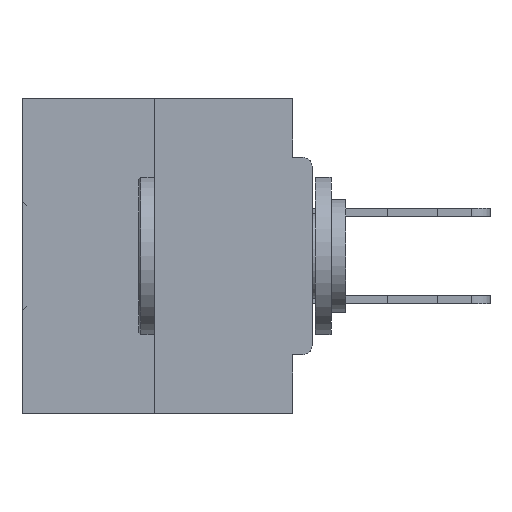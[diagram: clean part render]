
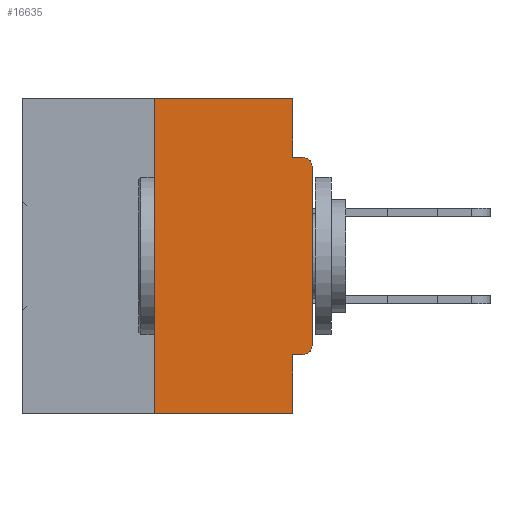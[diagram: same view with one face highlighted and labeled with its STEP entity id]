
A CAD part, left-side view. The second image highlights one B-rep face of the part: STEP entity #16635.
In plain terms, the highlighted planar face has unit normal (-1, 0, 0).
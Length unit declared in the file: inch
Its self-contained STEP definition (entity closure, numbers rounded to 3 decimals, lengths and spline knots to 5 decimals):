
#239 = VERTEX_POINT ( 'NONE', #18586 ) ;
#442 = VECTOR ( 'NONE', #19045, 39.37008 ) ;
#1625 = FACE_OUTER_BOUND ( 'NONE', #19300, .T. ) ;
#1790 = DIRECTION ( 'NONE',  ( 0., -1., 0. ) ) ;
#2994 = DIRECTION ( 'NONE',  ( 0., -1., 0. ) ) ;
#3037 = ORIENTED_EDGE ( 'NONE', *, *, #3227, .T. ) ;
#3147 = CARTESIAN_POINT ( 'NONE',  ( 0., 0.015, -0.4065 ) ) ;
#3227 = EDGE_CURVE ( 'NONE', #5612, #7826, #10813, .T. ) ;
#3352 = VECTOR ( 'NONE', #39458, 39.37008 ) ;
#4284 = CARTESIAN_POINT ( 'NONE',  ( 0., 0.25, 0. ) ) ;
#4488 = CARTESIAN_POINT ( 'NONE',  ( 0., 0.25, -0.5 ) ) ;
#4504 = LINE ( 'NONE', #40406, #442 ) ;
#4507 = AXIS2_PLACEMENT_3D ( 'NONE', #10167, #28764, #24775 ) ;
#5444 = LINE ( 'NONE', #20896, #45046 ) ;
#5584 = ORIENTED_EDGE ( 'NONE', *, *, #29936, .T. ) ;
#5612 = VERTEX_POINT ( 'NONE', #4488 ) ;
#6881 = LINE ( 'NONE', #23424, #43581 ) ;
#7826 = VERTEX_POINT ( 'NONE', #43231 ) ;
#8266 = ORIENTED_EDGE ( 'NONE', *, *, #36884, .T. ) ;
#9580 = VECTOR ( 'NONE', #22612, 39.37008 ) ;
#10167 = CARTESIAN_POINT ( 'NONE',  ( 0., 0.46, 0. ) ) ;
#10813 = LINE ( 'NONE', #12649, #36668 ) ;
#12649 = CARTESIAN_POINT ( 'NONE',  ( 0., 0.46, -0.5 ) ) ;
#12900 = VERTEX_POINT ( 'NONE', #28956 ) ;
#15367 = CARTESIAN_POINT ( 'NONE',  ( 0., 0.031, -0.5 ) ) ;
#16208 = LINE ( 'NONE', #46925, #29910 ) ;
#16635 = ADVANCED_FACE ( 'NONE', ( #1625 ), #39859, .F. ) ;
#17139 = CARTESIAN_POINT ( 'NONE',  ( 0., 0., -0.1085 ) ) ;
#17204 = AXIS2_PLACEMENT_3D ( 'NONE', #42694, #28243, #31471 ) ;
#18361 = DIRECTION ( 'NONE',  ( 0., 0., -1. ) ) ;
#18586 = CARTESIAN_POINT ( 'NONE',  ( 0., 0., -0.3915 ) ) ;
#19045 = DIRECTION ( 'NONE',  ( 0., 0., 1. ) ) ;
#19300 = EDGE_LOOP ( 'NONE', ( #36694, #38656, #3037, #40947, #28235, #27620, #5584, #8266, #20617, #40931 ) ) ;
#20617 = ORIENTED_EDGE ( 'NONE', *, *, #46822, .F. ) ;
#20896 = CARTESIAN_POINT ( 'NONE',  ( 0., 0.25, 0. ) ) ;
#21068 = CARTESIAN_POINT ( 'NONE',  ( 0., 0.031, -0.4065 ) ) ;
#22298 = CIRCLE ( 'NONE', #34668, 0.015 ) ;
#22612 = DIRECTION ( 'NONE',  ( 0., 0., -1. ) ) ;
#23424 = CARTESIAN_POINT ( 'NONE',  ( 0., 0., -0.0935 ) ) ;
#24067 = DIRECTION ( 'NONE',  ( 0., -1., 0. ) ) ;
#24616 = EDGE_CURVE ( 'NONE', #45241, #7826, #30230, .T. ) ;
#24775 = DIRECTION ( 'NONE',  ( 0., 0., -1. ) ) ;
#27364 = EDGE_CURVE ( 'NONE', #33543, #47430, #16208, .T. ) ;
#27620 = ORIENTED_EDGE ( 'NONE', *, *, #30322, .T. ) ;
#28095 = VERTEX_POINT ( 'NONE', #17139 ) ;
#28235 = ORIENTED_EDGE ( 'NONE', *, *, #29816, .F. ) ;
#28243 = DIRECTION ( 'NONE',  ( -1., 0., 0. ) ) ;
#28764 = DIRECTION ( 'NONE',  ( 1., 0., 0. ) ) ;
#28956 = CARTESIAN_POINT ( 'NONE',  ( 0., 0.015, -0.0935 ) ) ;
#29210 = VERTEX_POINT ( 'NONE', #3147 ) ;
#29816 = EDGE_CURVE ( 'NONE', #29210, #45241, #44090, .T. ) ;
#29910 = VECTOR ( 'NONE', #2994, 39.37008 ) ;
#29936 = EDGE_CURVE ( 'NONE', #239, #28095, #4504, .T. ) ;
#30230 = LINE ( 'NONE', #15367, #9580 ) ;
#30322 = EDGE_CURVE ( 'NONE', #29210, #239, #41180, .T. ) ;
#31388 = LINE ( 'NONE', #34684, #38308 ) ;
#31471 = DIRECTION ( 'NONE',  ( 0., 0., -1. ) ) ;
#31506 = DIRECTION ( 'NONE',  ( 0., 0., 1. ) ) ;
#32806 = EDGE_CURVE ( 'NONE', #5612, #33543, #5444, .T. ) ;
#32844 = CARTESIAN_POINT ( 'NONE',  ( 0., 0.015, -0.1085 ) ) ;
#33318 = DIRECTION ( 'NONE',  ( -1., 0., 0. ) ) ;
#33543 = VERTEX_POINT ( 'NONE', #4284 ) ;
#34668 = AXIS2_PLACEMENT_3D ( 'NONE', #32844, #33318, #18361 ) ;
#34684 = CARTESIAN_POINT ( 'NONE',  ( 0., 0.031, 0. ) ) ;
#34983 = CARTESIAN_POINT ( 'NONE',  ( 0., 0., -0.4065 ) ) ;
#36668 = VECTOR ( 'NONE', #24067, 39.37008 ) ;
#36694 = ORIENTED_EDGE ( 'NONE', *, *, #27364, .F. ) ;
#36884 = EDGE_CURVE ( 'NONE', #28095, #12900, #22298, .T. ) ;
#38308 = VECTOR ( 'NONE', #42507, 39.37008 ) ;
#38442 = CARTESIAN_POINT ( 'NONE',  ( 0., 0.031, -0.0935 ) ) ;
#38656 = ORIENTED_EDGE ( 'NONE', *, *, #32806, .F. ) ;
#38924 = EDGE_CURVE ( 'NONE', #47430, #45047, #31388, .T. ) ;
#39458 = DIRECTION ( 'NONE',  ( 0., 1., 0. ) ) ;
#39859 = PLANE ( 'NONE',  #4507 ) ;
#40406 = CARTESIAN_POINT ( 'NONE',  ( 0., 0., 0. ) ) ;
#40931 = ORIENTED_EDGE ( 'NONE', *, *, #38924, .F. ) ;
#40947 = ORIENTED_EDGE ( 'NONE', *, *, #24616, .F. ) ;
#41180 = CIRCLE ( 'NONE', #17204, 0.015 ) ;
#42507 = DIRECTION ( 'NONE',  ( 0., 0., -1. ) ) ;
#42694 = CARTESIAN_POINT ( 'NONE',  ( 0., 0.015, -0.3915 ) ) ;
#43231 = CARTESIAN_POINT ( 'NONE',  ( 0., 0.031, -0.5 ) ) ;
#43581 = VECTOR ( 'NONE', #1790, 39.37008 ) ;
#44090 = LINE ( 'NONE', #34983, #3352 ) ;
#45046 = VECTOR ( 'NONE', #31506, 39.37008 ) ;
#45047 = VERTEX_POINT ( 'NONE', #38442 ) ;
#45241 = VERTEX_POINT ( 'NONE', #21068 ) ;
#46822 = EDGE_CURVE ( 'NONE', #45047, #12900, #6881, .T. ) ;
#46925 = CARTESIAN_POINT ( 'NONE',  ( 0., 0.46, 0. ) ) ;
#47212 = CARTESIAN_POINT ( 'NONE',  ( 0., 0.031, 0. ) ) ;
#47430 = VERTEX_POINT ( 'NONE', #47212 ) ;
